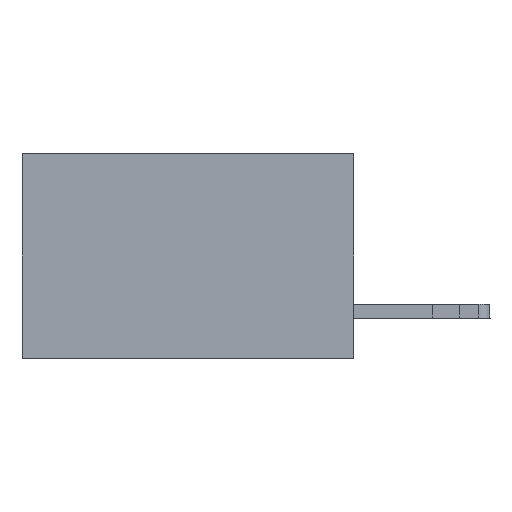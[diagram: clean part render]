
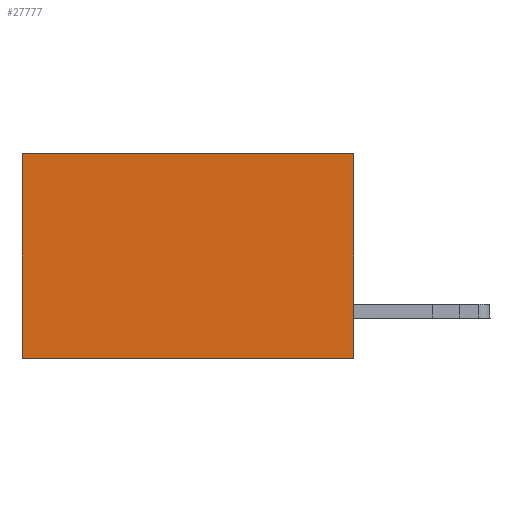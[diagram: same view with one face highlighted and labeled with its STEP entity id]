
A CAD part, left-side view. The second image highlights one B-rep face of the part: STEP entity #27777.
In plain terms, the highlighted planar face has unit normal (-1, 0, 0).
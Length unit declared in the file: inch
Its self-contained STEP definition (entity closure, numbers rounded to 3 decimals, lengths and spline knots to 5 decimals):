
#97 = CARTESIAN_POINT ( 'NONE',  ( 0.2875, 0., 0. ) ) ;
#908 = LINE ( 'NONE', #28692, #28409 ) ;
#1477 = DIRECTION ( 'NONE',  ( 0., 1., 0. ) ) ;
#2104 = CARTESIAN_POINT ( 'NONE',  ( 0.2875, 0.6, 0. ) ) ;
#2165 = VERTEX_POINT ( 'NONE', #2104 ) ;
#2293 = VECTOR ( 'NONE', #1477, 39.37008 ) ;
#3210 = CARTESIAN_POINT ( 'NONE',  ( 0.2875, 0.6, 0. ) ) ;
#3218 = EDGE_CURVE ( 'NONE', #10977, #2165, #908, .T. ) ;
#4021 = CARTESIAN_POINT ( 'NONE',  ( 0.2875, 0., -0.37 ) ) ;
#4023 = VECTOR ( 'NONE', #25816, 39.37008 ) ;
#4796 = LINE ( 'NONE', #3210, #4023 ) ;
#6786 = ORIENTED_EDGE ( 'NONE', *, *, #7967, .F. ) ;
#7579 = CARTESIAN_POINT ( 'NONE',  ( 0.2875, 0., 0. ) ) ;
#7908 = CARTESIAN_POINT ( 'NONE',  ( 0.2875, 0.6, -0.37 ) ) ;
#7967 = EDGE_CURVE ( 'NONE', #18979, #31296, #9035, .T. ) ;
#8324 = CARTESIAN_POINT ( 'NONE',  ( 0.2875, 0., -0.37 ) ) ;
#9035 = LINE ( 'NONE', #4021, #2293 ) ;
#10359 = CARTESIAN_POINT ( 'NONE',  ( 0.2875, 0., 0. ) ) ;
#10977 = VERTEX_POINT ( 'NONE', #10359 ) ;
#11471 = FACE_OUTER_BOUND ( 'NONE', #13430, .T. ) ;
#11986 = VECTOR ( 'NONE', #17847, 39.37008 ) ;
#12260 = EDGE_CURVE ( 'NONE', #2165, #31296, #4796, .T. ) ;
#12774 = LINE ( 'NONE', #97, #11986 ) ;
#13221 = ORIENTED_EDGE ( 'NONE', *, *, #13248, .F. ) ;
#13241 = DIRECTION ( 'NONE',  ( 1., 0., 0. ) ) ;
#13248 = EDGE_CURVE ( 'NONE', #10977, #18979, #12774, .T. ) ;
#13430 = EDGE_LOOP ( 'NONE', ( #19110, #6786, #13221, #21255 ) ) ;
#15250 = PLANE ( 'NONE',  #20012 ) ;
#17754 = DIRECTION ( 'NONE',  ( 0., 0., -1. ) ) ;
#17847 = DIRECTION ( 'NONE',  ( 0., 0., -1. ) ) ;
#18979 = VERTEX_POINT ( 'NONE', #8324 ) ;
#19110 = ORIENTED_EDGE ( 'NONE', *, *, #12260, .T. ) ;
#20012 = AXIS2_PLACEMENT_3D ( 'NONE', #7579, #13241, #17754 ) ;
#21255 = ORIENTED_EDGE ( 'NONE', *, *, #3218, .T. ) ;
#23919 = DIRECTION ( 'NONE',  ( 0., 1., 0. ) ) ;
#25816 = DIRECTION ( 'NONE',  ( 0., 0., -1. ) ) ;
#27777 = ADVANCED_FACE ( 'NONE', ( #11471 ), #15250, .F. ) ;
#28409 = VECTOR ( 'NONE', #23919, 39.37008 ) ;
#28692 = CARTESIAN_POINT ( 'NONE',  ( 0.2875, 0., 0. ) ) ;
#31296 = VERTEX_POINT ( 'NONE', #7908 ) ;
